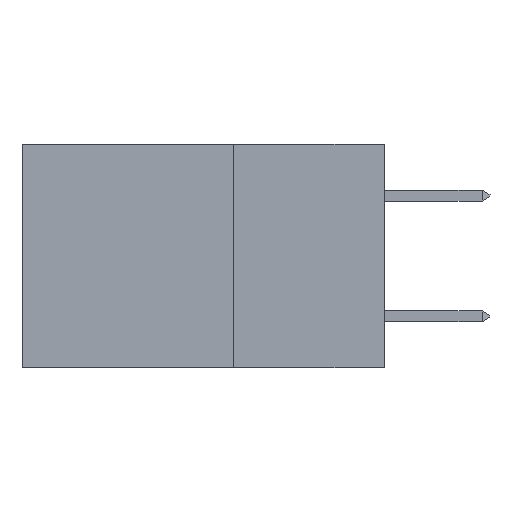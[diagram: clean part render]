
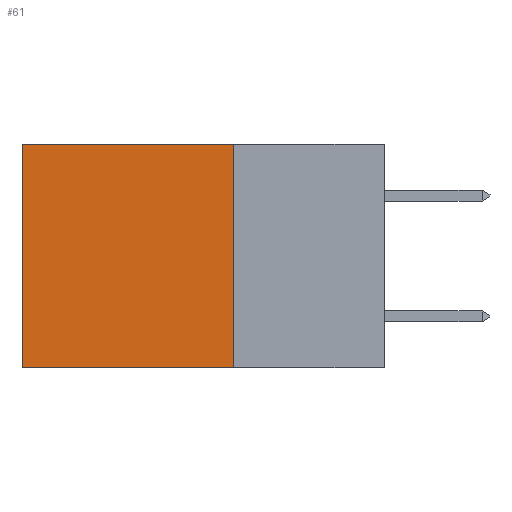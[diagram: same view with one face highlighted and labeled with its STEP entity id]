
A CAD part, left-side view. The second image highlights one B-rep face of the part: STEP entity #61.
In plain terms, the highlighted planar face has unit normal (-1, 0, 0).
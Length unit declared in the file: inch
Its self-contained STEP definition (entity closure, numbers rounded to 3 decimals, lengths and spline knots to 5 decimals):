
#61 = ADVANCED_FACE ( 'NONE', ( #3169 ), #7878, .F. ) ;
#175 = DIRECTION ( 'NONE',  ( 0., 1., 0. ) ) ;
#202 = EDGE_CURVE ( 'NONE', #7610, #19506, #13861, .T. ) ;
#254 = CARTESIAN_POINT ( 'NONE',  ( 0.2875, 0.6, 0. ) ) ;
#445 = DIRECTION ( 'NONE',  ( 0., 0., -1. ) ) ;
#1814 = CARTESIAN_POINT ( 'NONE',  ( 0.2875, 0.25, -0.37 ) ) ;
#3169 = FACE_OUTER_BOUND ( 'NONE', #20088, .T. ) ;
#4365 = CARTESIAN_POINT ( 'NONE',  ( 0.2875, 0.25, 0. ) ) ;
#4497 = LINE ( 'NONE', #20202, #20693 ) ;
#5144 = VECTOR ( 'NONE', #175, 39.37008 ) ;
#6014 = CARTESIAN_POINT ( 'NONE',  ( 0.2875, 0.25, 0. ) ) ;
#6601 = CARTESIAN_POINT ( 'NONE',  ( 0.2875, 0.6, 0. ) ) ;
#7058 = ORIENTED_EDGE ( 'NONE', *, *, #17248, .F. ) ;
#7508 = CARTESIAN_POINT ( 'NONE',  ( 0.2875, 0.25, 0. ) ) ;
#7610 = VERTEX_POINT ( 'NONE', #6014 ) ;
#7878 = PLANE ( 'NONE',  #12064 ) ;
#10152 = DIRECTION ( 'NONE',  ( 0., 0., -1. ) ) ;
#10675 = ORIENTED_EDGE ( 'NONE', *, *, #11497, .T. ) ;
#10949 = ORIENTED_EDGE ( 'NONE', *, *, #19455, .F. ) ;
#11497 = EDGE_CURVE ( 'NONE', #19506, #17450, #18066, .T. ) ;
#11909 = CARTESIAN_POINT ( 'NONE',  ( 0.2875, 0.6, -0.37 ) ) ;
#12064 = AXIS2_PLACEMENT_3D ( 'NONE', #4365, #12843, #445 ) ;
#12843 = DIRECTION ( 'NONE',  ( 1., 0., 0. ) ) ;
#13394 = VECTOR ( 'NONE', #13439, 39.37008 ) ;
#13439 = DIRECTION ( 'NONE',  ( 0., 1., 0. ) ) ;
#13861 = LINE ( 'NONE', #7508, #13394 ) ;
#14188 = VECTOR ( 'NONE', #10152, 39.37008 ) ;
#14414 = DIRECTION ( 'NONE',  ( 0., 0., -1. ) ) ;
#17248 = EDGE_CURVE ( 'NONE', #7610, #18216, #4497, .T. ) ;
#17450 = VERTEX_POINT ( 'NONE', #11909 ) ;
#17869 = LINE ( 'NONE', #19512, #5144 ) ;
#18066 = LINE ( 'NONE', #6601, #14188 ) ;
#18216 = VERTEX_POINT ( 'NONE', #1814 ) ;
#18875 = ORIENTED_EDGE ( 'NONE', *, *, #202, .T. ) ;
#19455 = EDGE_CURVE ( 'NONE', #18216, #17450, #17869, .T. ) ;
#19506 = VERTEX_POINT ( 'NONE', #254 ) ;
#19512 = CARTESIAN_POINT ( 'NONE',  ( 0.2875, 0.25, -0.37 ) ) ;
#20088 = EDGE_LOOP ( 'NONE', ( #10675, #10949, #7058, #18875 ) ) ;
#20202 = CARTESIAN_POINT ( 'NONE',  ( 0.2875, 0.25, 0. ) ) ;
#20693 = VECTOR ( 'NONE', #14414, 39.37008 ) ;
